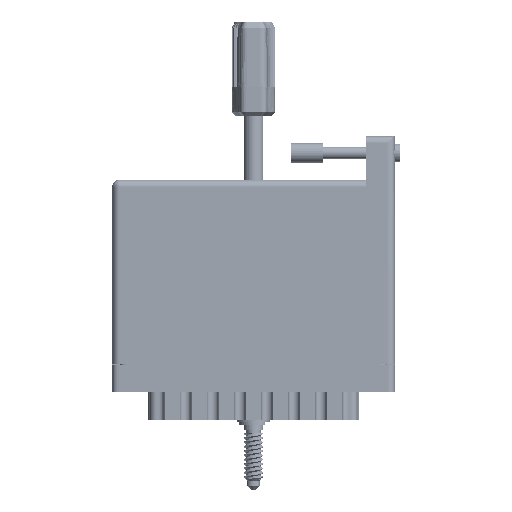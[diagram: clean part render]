
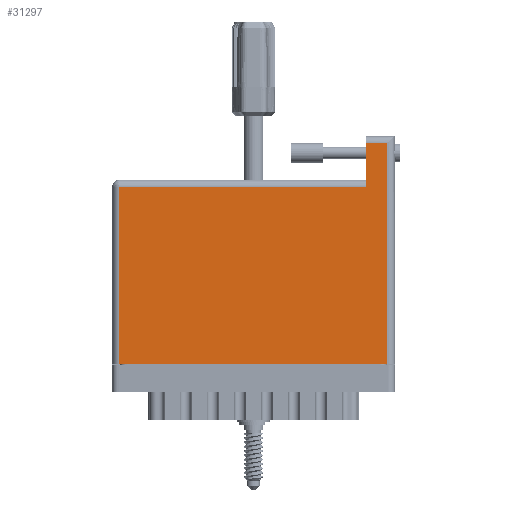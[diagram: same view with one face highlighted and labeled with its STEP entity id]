
A CAD part, front view. The second image highlights one B-rep face of the part: STEP entity #31297.
In plain terms, the highlighted face is planar.
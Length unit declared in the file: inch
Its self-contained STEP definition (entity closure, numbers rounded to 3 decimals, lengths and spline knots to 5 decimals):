
#1466 = VERTEX_POINT ( 'NONE', #86778 ) ;
#5687 = CARTESIAN_POINT ( 'NONE',  ( 0.07, 0., 0. ) ) ;
#6013 = VERTEX_POINT ( 'NONE', #15167 ) ;
#6117 = DIRECTION ( 'NONE',  ( 0., 0., -1. ) ) ;
#13660 = CARTESIAN_POINT ( 'NONE',  ( 2.438, 1.705, 0. ) ) ;
#13911 = LINE ( 'NONE', #20711, #67547 ) ;
#15167 = CARTESIAN_POINT ( 'NONE',  ( 2.648, 0., 0. ) ) ;
#15482 = ORIENTED_EDGE ( 'NONE', *, *, #31307, .T. ) ;
#19233 = VECTOR ( 'NONE', #32815, 39.37008 ) ;
#20612 = CARTESIAN_POINT ( 'NONE',  ( 2.438, 2.195, 0. ) ) ;
#20703 = CARTESIAN_POINT ( 'NONE',  ( 0.07, 0., 0. ) ) ;
#20711 = CARTESIAN_POINT ( 'NONE',  ( 0., 1.705, 0. ) ) ;
#25420 = EDGE_CURVE ( 'NONE', #33145, #73913, #61673, .T. ) ;
#26475 = VECTOR ( 'NONE', #77785, 39.37008 ) ;
#26721 = EDGE_CURVE ( 'NONE', #75610, #45401, #60786, .T. ) ;
#27389 = PLANE ( 'NONE',  #58143 ) ;
#31297 = ADVANCED_FACE ( 'NONE', ( #75229 ), #27389, .F. ) ;
#31307 = EDGE_CURVE ( 'NONE', #6013, #1466, #54908, .T. ) ;
#31922 = EDGE_CURVE ( 'NONE', #1466, #33145, #84573, .T. ) ;
#32381 = DIRECTION ( 'NONE',  ( 0., -1., 0. ) ) ;
#32815 = DIRECTION ( 'NONE',  ( 0., 1., 0. ) ) ;
#33145 = VERTEX_POINT ( 'NONE', #46692 ) ;
#33257 = CARTESIAN_POINT ( 'NONE',  ( 0., 1.775, 0. ) ) ;
#38906 = ORIENTED_EDGE ( 'NONE', *, *, #25420, .T. ) ;
#40648 = ORIENTED_EDGE ( 'NONE', *, *, #26721, .T. ) ;
#41355 = DIRECTION ( 'NONE',  ( 0., -1., 0. ) ) ;
#45401 = VERTEX_POINT ( 'NONE', #20703 ) ;
#45896 = EDGE_CURVE ( 'NONE', #45401, #6013, #51096, .T. ) ;
#46692 = CARTESIAN_POINT ( 'NONE',  ( 2.438, 2.125, 0. ) ) ;
#48119 = CARTESIAN_POINT ( 'NONE',  ( 2.648, 2.195, 0. ) ) ;
#49029 = EDGE_CURVE ( 'NONE', #73913, #75610, #13911, .T. ) ;
#49169 = EDGE_LOOP ( 'NONE', ( #51432, #40648, #52972, #15482, #67922, #38906 ) ) ;
#51096 = LINE ( 'NONE', #78642, #60184 ) ;
#51432 = ORIENTED_EDGE ( 'NONE', *, *, #49029, .T. ) ;
#52972 = ORIENTED_EDGE ( 'NONE', *, *, #45896, .T. ) ;
#54024 = DIRECTION ( 'NONE',  ( -1., 0., 0. ) ) ;
#54908 = LINE ( 'NONE', #48119, #19233 ) ;
#58143 = AXIS2_PLACEMENT_3D ( 'NONE', #33257, #6117, #54024 ) ;
#60184 = VECTOR ( 'NONE', #71860, 39.37008 ) ;
#60786 = LINE ( 'NONE', #5687, #76215 ) ;
#61673 = LINE ( 'NONE', #20612, #83190 ) ;
#67547 = VECTOR ( 'NONE', #82123, 39.37008 ) ;
#67922 = ORIENTED_EDGE ( 'NONE', *, *, #31922, .T. ) ;
#71860 = DIRECTION ( 'NONE',  ( 1., 0., 0. ) ) ;
#73913 = VERTEX_POINT ( 'NONE', #13660 ) ;
#75229 = FACE_OUTER_BOUND ( 'NONE', #49169, .T. ) ;
#75610 = VERTEX_POINT ( 'NONE', #84404 ) ;
#76006 = CARTESIAN_POINT ( 'NONE',  ( 0., 2.125, 0. ) ) ;
#76215 = VECTOR ( 'NONE', #32381, 39.37008 ) ;
#77785 = DIRECTION ( 'NONE',  ( -1., 0., 0. ) ) ;
#78642 = CARTESIAN_POINT ( 'NONE',  ( 0., 0., 0. ) ) ;
#82123 = DIRECTION ( 'NONE',  ( -1., 0., 0. ) ) ;
#83190 = VECTOR ( 'NONE', #41355, 39.37008 ) ;
#84404 = CARTESIAN_POINT ( 'NONE',  ( 0.07, 1.705, 0. ) ) ;
#84573 = LINE ( 'NONE', #76006, #26475 ) ;
#86778 = CARTESIAN_POINT ( 'NONE',  ( 2.648, 2.125, 0. ) ) ;
